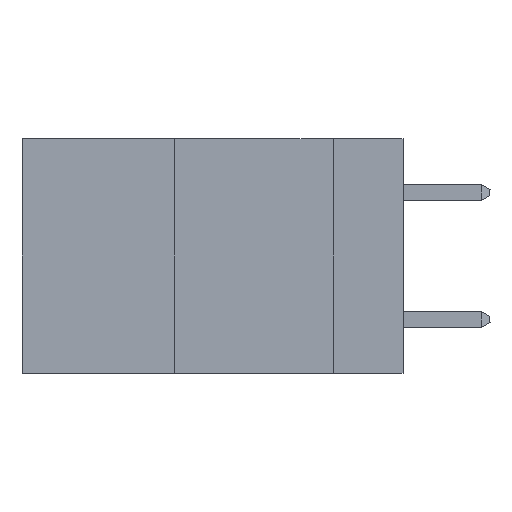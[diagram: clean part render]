
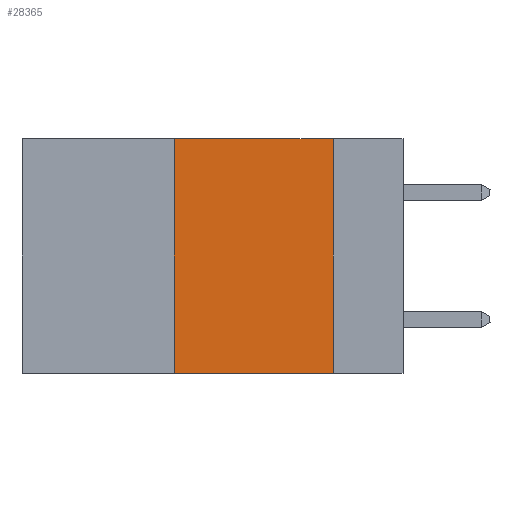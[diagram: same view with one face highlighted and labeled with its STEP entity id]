
A CAD part, left-side view. The second image highlights one B-rep face of the part: STEP entity #28365.
In plain terms, the highlighted planar face has unit normal (-1, 0, 0).
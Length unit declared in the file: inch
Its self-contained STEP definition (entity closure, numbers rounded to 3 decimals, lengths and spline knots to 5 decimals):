
#543 = DIRECTION ( 'NONE',  ( 1., 0., 0. ) ) ;
#1305 = EDGE_LOOP ( 'NONE', ( #11375, #3628, #28735, #36490 ) ) ;
#1370 = AXIS2_PLACEMENT_3D ( 'NONE', #33551, #543, #41046 ) ;
#1408 = VERTEX_POINT ( 'NONE', #5145 ) ;
#2963 = LINE ( 'NONE', #30499, #32197 ) ;
#3628 = ORIENTED_EDGE ( 'NONE', *, *, #20244, .F. ) ;
#3739 = CARTESIAN_POINT ( 'NONE',  ( 0., 0.11, 0. ) ) ;
#5145 = CARTESIAN_POINT ( 'NONE',  ( 0., 0.11, 0. ) ) ;
#6269 = CARTESIAN_POINT ( 'NONE',  ( 0., 0.36, -0.37 ) ) ;
#6283 = CARTESIAN_POINT ( 'NONE',  ( 0., 0.11, -0.37 ) ) ;
#11375 = ORIENTED_EDGE ( 'NONE', *, *, #32716, .F. ) ;
#12994 = VECTOR ( 'NONE', #23388, 39.37008 ) ;
#15705 = CARTESIAN_POINT ( 'NONE',  ( 0., 0.36, 0. ) ) ;
#17807 = FACE_OUTER_BOUND ( 'NONE', #1305, .T. ) ;
#19538 = VECTOR ( 'NONE', #41799, 39.37008 ) ;
#19562 = DIRECTION ( 'NONE',  ( 0., -1., 0. ) ) ;
#20244 = EDGE_CURVE ( 'NONE', #46948, #1408, #42485, .T. ) ;
#21040 = VERTEX_POINT ( 'NONE', #6269 ) ;
#22643 = EDGE_CURVE ( 'NONE', #21040, #46948, #27300, .T. ) ;
#22780 = PLANE ( 'NONE',  #1370 ) ;
#23388 = DIRECTION ( 'NONE',  ( 0., 0., 1. ) ) ;
#25274 = EDGE_CURVE ( 'NONE', #21040, #42395, #2963, .T. ) ;
#27300 = LINE ( 'NONE', #15705, #12994 ) ;
#28365 = ADVANCED_FACE ( 'NONE', ( #17807 ), #22780, .F. ) ;
#28506 = VECTOR ( 'NONE', #33385, 39.37008 ) ;
#28735 = ORIENTED_EDGE ( 'NONE', *, *, #22643, .F. ) ;
#30499 = CARTESIAN_POINT ( 'NONE',  ( 0., 0.6, -0.37 ) ) ;
#32197 = VECTOR ( 'NONE', #19562, 39.37008 ) ;
#32716 = EDGE_CURVE ( 'NONE', #1408, #42395, #33675, .T. ) ;
#33385 = DIRECTION ( 'NONE',  ( 0., 0., -1. ) ) ;
#33551 = CARTESIAN_POINT ( 'NONE',  ( 0., 0.6, 0. ) ) ;
#33675 = LINE ( 'NONE', #3739, #28506 ) ;
#36490 = ORIENTED_EDGE ( 'NONE', *, *, #25274, .T. ) ;
#40430 = CARTESIAN_POINT ( 'NONE',  ( 0., 0.36, 0. ) ) ;
#41046 = DIRECTION ( 'NONE',  ( 0., 0., -1. ) ) ;
#41799 = DIRECTION ( 'NONE',  ( 0., -1., 0. ) ) ;
#42395 = VERTEX_POINT ( 'NONE', #6283 ) ;
#42485 = LINE ( 'NONE', #45155, #19538 ) ;
#45155 = CARTESIAN_POINT ( 'NONE',  ( 0., 0.6, 0. ) ) ;
#46948 = VERTEX_POINT ( 'NONE', #40430 ) ;
